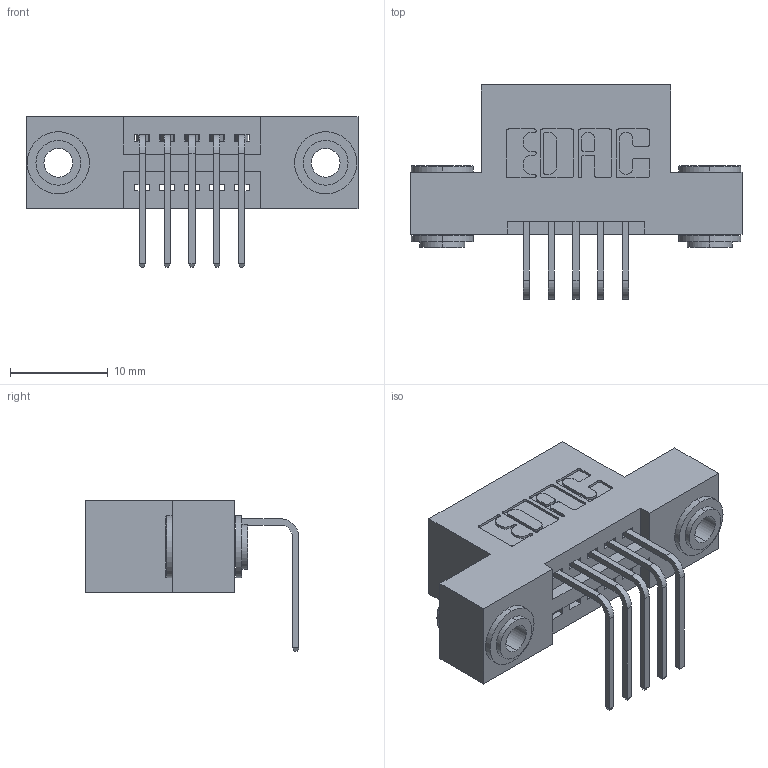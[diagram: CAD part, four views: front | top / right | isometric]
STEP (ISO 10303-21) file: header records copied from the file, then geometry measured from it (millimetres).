
FILE_DESCRIPTION (( 'STEP AP203' ), '1' );
FILE_NAME ('395-005-558-103.STEP', '2018-10-23T18:37:02', ( '' ), ( '' ), 'SwSTEP 2.0', 'SolidWorks 2016', '' );
FILE_SCHEMA (( 'CONFIG_CONTROL_DESIGN' ));
Length unit declared in the file: inch
Products named in the file (4): 345 Part_Flush Mounting Lugs - 0.156 Dia-TH; 395-005-558-103; 345-292-001_558 Tail - 2; 345-250-002_345-250-002-102
Assembly tree (8 placements, depth 2):
  395-005-558-103
    345 Part_Flush Mounting Lugs - 0.156 Dia-TH
    345-292-001_558 Tail - 2  x5
    345-250-002_345-250-002-102  x2
Bounding box: 33.91 x 21.83 x 15.37 mm (x, y, z)
Volume: 2953.7 mm3; surface area: 3734.7 mm2
Topology: 8 solids, 8 shells, 464 faces, 1327 edges, 874 vertices
Faces by surface type: plane 300, cylinder 156, cone 8
Entity records: 9478 total; most frequent: CARTESIAN_POINT 1622, ORIENTED_EDGE 1554, DIRECTION 1501, EDGE_CURVE 777, VECTOR 601, LINE 601, VERTEX_POINT 514, AXIS2_PLACEMENT_3D 450
